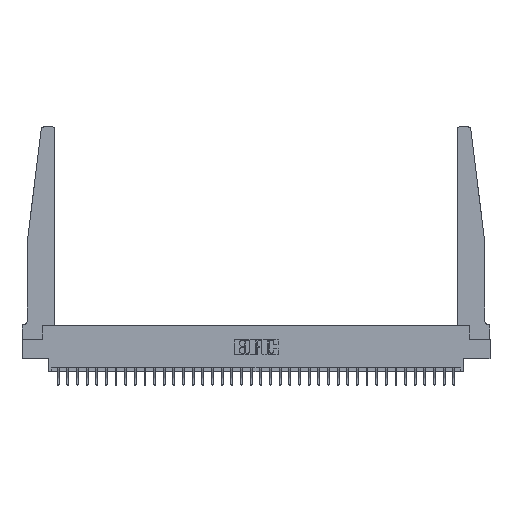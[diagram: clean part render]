
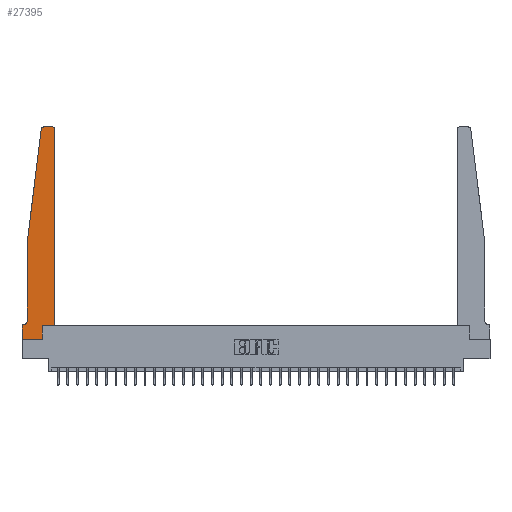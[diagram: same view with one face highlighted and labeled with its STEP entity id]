
A CAD part, top view. The second image highlights one B-rep face of the part: STEP entity #27395.
In plain terms, the highlighted planar face has unit normal (0, 0, 1).
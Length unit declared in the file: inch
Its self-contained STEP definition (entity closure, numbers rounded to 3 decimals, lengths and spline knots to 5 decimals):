
#25 = VECTOR ( 'NONE', #20112, 39.37008 ) ;
#593 = EDGE_CURVE ( 'NONE', #9248, #7443, #28675, .T. ) ;
#909 = AXIS2_PLACEMENT_3D ( 'NONE', #26004, #10957, #28547 ) ;
#1442 = FACE_OUTER_BOUND ( 'NONE', #11499, .T. ) ;
#1697 = CARTESIAN_POINT ( 'NONE',  ( 0.2605, 0., 0.37 ) ) ;
#1948 = ORIENTED_EDGE ( 'NONE', *, *, #20144, .T. ) ;
#2329 = DIRECTION ( 'NONE',  ( 0., 0., 1. ) ) ;
#2653 = EDGE_CURVE ( 'NONE', #30965, #18549, #26180, .T. ) ;
#2856 = CARTESIAN_POINT ( 'NONE',  ( 0.2605, 0.18, 0.37 ) ) ;
#2927 = ORIENTED_EDGE ( 'NONE', *, *, #25831, .T. ) ;
#2945 = DIRECTION ( 'NONE',  ( 1., 0., 0. ) ) ;
#3204 = VERTEX_POINT ( 'NONE', #23462 ) ;
#3410 = DIRECTION ( 'NONE',  ( -1., 0., 0. ) ) ;
#3930 = ORIENTED_EDGE ( 'NONE', *, *, #28539, .T. ) ;
#4399 = CARTESIAN_POINT ( 'NONE',  ( 0., 0., 0.37 ) ) ;
#4421 = DIRECTION ( 'NONE',  ( 1., 0., 0. ) ) ;
#5536 = CARTESIAN_POINT ( 'NONE',  ( 0.425, 0.18, 0.37 ) ) ;
#5960 = AXIS2_PLACEMENT_3D ( 'NONE', #17378, #2329, #19909 ) ;
#6076 = VERTEX_POINT ( 'NONE', #16536 ) ;
#6119 = DIRECTION ( 'NONE',  ( 0., -1., 0. ) ) ;
#6167 = AXIS2_PLACEMENT_3D ( 'NONE', #14441, #19475, #4421 ) ;
#6412 = CARTESIAN_POINT ( 'NONE',  ( 0.25, 2.75, 0.37 ) ) ;
#6655 = CARTESIAN_POINT ( 'NONE',  ( 0., 0.1875, 0.37 ) ) ;
#7313 = DIRECTION ( 'NONE',  ( -0.122, -0.992, 0. ) ) ;
#7443 = VERTEX_POINT ( 'NONE', #9233 ) ;
#8091 = LINE ( 'NONE', #25589, #26573 ) ;
#8377 = CARTESIAN_POINT ( 'NONE',  ( 0.065, 0.1875, 0.37 ) ) ;
#9233 = CARTESIAN_POINT ( 'NONE',  ( 0.395, 2.75, 0.37 ) ) ;
#9248 = VERTEX_POINT ( 'NONE', #14385 ) ;
#9767 = CARTESIAN_POINT ( 'NONE',  ( 0.065, 1.25, 0.37 ) ) ;
#9785 = EDGE_CURVE ( 'NONE', #7443, #19583, #25128, .T. ) ;
#10957 = DIRECTION ( 'NONE',  ( 0., 0., 1. ) ) ;
#11013 = VECTOR ( 'NONE', #30630, 39.37008 ) ;
#11499 = EDGE_LOOP ( 'NONE', ( #15537, #3930, #13874, #18163, #2927, #17456, #25694, #1948, #12520, #15303, #19408, #16259 ) ) ;
#11755 = VECTOR ( 'NONE', #24023, 39.37008 ) ;
#12520 = ORIENTED_EDGE ( 'NONE', *, *, #13175, .T. ) ;
#12682 = VERTEX_POINT ( 'NONE', #26182 ) ;
#13175 = EDGE_CURVE ( 'NONE', #22852, #30698, #13704, .T. ) ;
#13268 = CARTESIAN_POINT ( 'NONE',  ( 0., 0., 0.37 ) ) ;
#13704 = LINE ( 'NONE', #2856, #26285 ) ;
#13779 = CARTESIAN_POINT ( 'NONE',  ( 0.015, 0.2375, 0.37 ) ) ;
#13874 = ORIENTED_EDGE ( 'NONE', *, *, #28771, .T. ) ;
#14361 = CIRCLE ( 'NONE', #909, 0.03 ) ;
#14385 = CARTESIAN_POINT ( 'NONE',  ( 0.425, 2.72, 0.37 ) ) ;
#14441 = CARTESIAN_POINT ( 'NONE',  ( 0., 0.1875, 0.37 ) ) ;
#14872 = EDGE_CURVE ( 'NONE', #30698, #19040, #8091, .T. ) ;
#15303 = ORIENTED_EDGE ( 'NONE', *, *, #14872, .T. ) ;
#15411 = VECTOR ( 'NONE', #3410, 39.37008 ) ;
#15537 = ORIENTED_EDGE ( 'NONE', *, *, #9785, .T. ) ;
#16053 = AXIS2_PLACEMENT_3D ( 'NONE', #13779, #31360, #16314 ) ;
#16259 = ORIENTED_EDGE ( 'NONE', *, *, #593, .T. ) ;
#16314 = DIRECTION ( 'NONE',  ( -1., 0., 0. ) ) ;
#16393 = VECTOR ( 'NONE', #24230, 39.37008 ) ;
#16536 = CARTESIAN_POINT ( 'NONE',  ( 0.24675, 2.72367, 0.37 ) ) ;
#16630 = CARTESIAN_POINT ( 'NONE',  ( 0.425, 0.18, 0.37 ) ) ;
#16942 = PLANE ( 'NONE',  #6167 ) ;
#17378 = CARTESIAN_POINT ( 'NONE',  ( 0.395, 2.72, 0.37 ) ) ;
#17456 = ORIENTED_EDGE ( 'NONE', *, *, #19832, .T. ) ;
#17894 = DIRECTION ( 'NONE',  ( 0., 1., 0. ) ) ;
#18163 = ORIENTED_EDGE ( 'NONE', *, *, #2653, .T. ) ;
#18549 = VERTEX_POINT ( 'NONE', #18770 ) ;
#18770 = CARTESIAN_POINT ( 'NONE',  ( 0.065, 0.2375, 0.37 ) ) ;
#19040 = VERTEX_POINT ( 'NONE', #5536 ) ;
#19408 = ORIENTED_EDGE ( 'NONE', *, *, #27313, .T. ) ;
#19475 = DIRECTION ( 'NONE',  ( 0., 0., 1. ) ) ;
#19583 = VERTEX_POINT ( 'NONE', #25213 ) ;
#19832 = EDGE_CURVE ( 'NONE', #3204, #20996, #29569, .T. ) ;
#19909 = DIRECTION ( 'NONE',  ( 1., 0., 0. ) ) ;
#20081 = LINE ( 'NONE', #4399, #25 ) ;
#20112 = DIRECTION ( 'NONE',  ( 1., 0., 0. ) ) ;
#20144 = EDGE_CURVE ( 'NONE', #12682, #22852, #20081, .T. ) ;
#20712 = EDGE_CURVE ( 'NONE', #20996, #12682, #31060, .T. ) ;
#20996 = VERTEX_POINT ( 'NONE', #6655 ) ;
#22222 = LINE ( 'NONE', #9767, #27314 ) ;
#22852 = VERTEX_POINT ( 'NONE', #1697 ) ;
#23097 = LINE ( 'NONE', #16630, #16393 ) ;
#23462 = CARTESIAN_POINT ( 'NONE',  ( 0.015, 0.1875, 0.37 ) ) ;
#23722 = CARTESIAN_POINT ( 'NONE',  ( 0.065, 1.25, 0.37 ) ) ;
#24023 = DIRECTION ( 'NONE',  ( -1., 0., 0. ) ) ;
#24230 = DIRECTION ( 'NONE',  ( 0., 1., 0. ) ) ;
#25128 = LINE ( 'NONE', #6412, #11755 ) ;
#25213 = CARTESIAN_POINT ( 'NONE',  ( 0.27653, 2.75, 0.37 ) ) ;
#25404 = VECTOR ( 'NONE', #6119, 39.37008 ) ;
#25589 = CARTESIAN_POINT ( 'NONE',  ( 0.425, 0.18, 0.37 ) ) ;
#25694 = ORIENTED_EDGE ( 'NONE', *, *, #20712, .T. ) ;
#25831 = EDGE_CURVE ( 'NONE', #18549, #3204, #30650, .T. ) ;
#26004 = CARTESIAN_POINT ( 'NONE',  ( 0.27653, 2.72, 0.37 ) ) ;
#26180 = LINE ( 'NONE', #23722, #25404 ) ;
#26182 = CARTESIAN_POINT ( 'NONE',  ( 0., 0., 0.37 ) ) ;
#26199 = CARTESIAN_POINT ( 'NONE',  ( 0.2605, 0.18, 0.37 ) ) ;
#26285 = VECTOR ( 'NONE', #17894, 39.37008 ) ;
#26573 = VECTOR ( 'NONE', #2945, 39.37008 ) ;
#27313 = EDGE_CURVE ( 'NONE', #19040, #9248, #23097, .T. ) ;
#27314 = VECTOR ( 'NONE', #7313, 39.37008 ) ;
#27395 = ADVANCED_FACE ( 'NONE', ( #1442 ), #16942, .T. ) ;
#28539 = EDGE_CURVE ( 'NONE', #19583, #6076, #14361, .T. ) ;
#28547 = DIRECTION ( 'NONE',  ( 1., 0., 0. ) ) ;
#28675 = CIRCLE ( 'NONE', #5960, 0.03 ) ;
#28771 = EDGE_CURVE ( 'NONE', #6076, #30965, #22222, .T. ) ;
#29569 = LINE ( 'NONE', #8377, #15411 ) ;
#29822 = CARTESIAN_POINT ( 'NONE',  ( 0.065, 1.25, 0.37 ) ) ;
#30630 = DIRECTION ( 'NONE',  ( 0., -1., 0. ) ) ;
#30650 = CIRCLE ( 'NONE', #16053, 0.05 ) ;
#30698 = VERTEX_POINT ( 'NONE', #26199 ) ;
#30965 = VERTEX_POINT ( 'NONE', #29822 ) ;
#31060 = LINE ( 'NONE', #13268, #11013 ) ;
#31360 = DIRECTION ( 'NONE',  ( 0., 0., -1. ) ) ;
